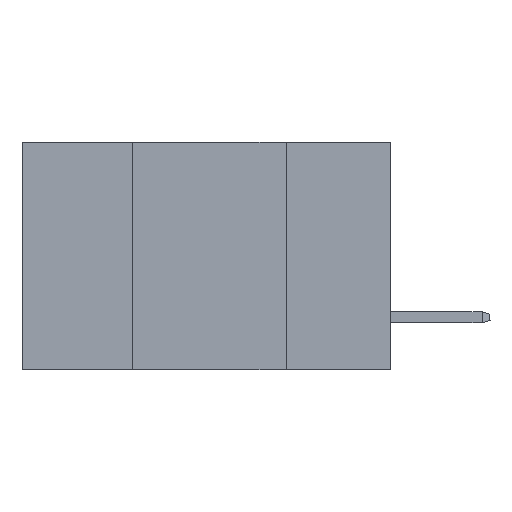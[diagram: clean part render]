
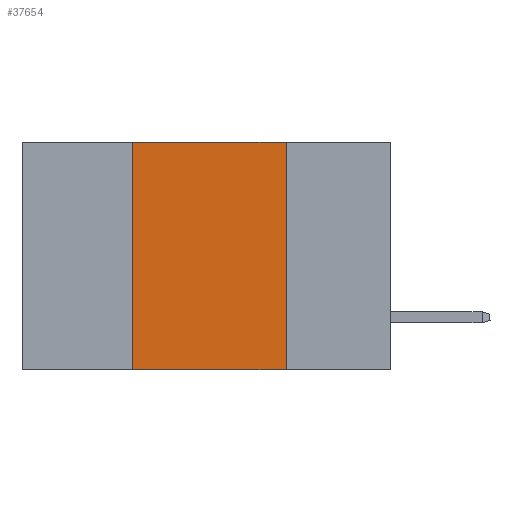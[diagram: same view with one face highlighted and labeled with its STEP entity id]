
A CAD part, left-side view. The second image highlights one B-rep face of the part: STEP entity #37654.
In plain terms, the highlighted planar face has unit normal (-1, 0, 0).
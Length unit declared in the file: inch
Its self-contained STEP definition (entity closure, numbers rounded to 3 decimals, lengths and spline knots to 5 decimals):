
#202 = CARTESIAN_POINT ( 'NONE',  ( 0., 0.17, -0.37 ) ) ;
#1221 = VERTEX_POINT ( 'NONE', #202 ) ;
#5939 = DIRECTION ( 'NONE',  ( 0., 0., 1. ) ) ;
#6066 = CARTESIAN_POINT ( 'NONE',  ( 0., 0.6, 0. ) ) ;
#6353 = LINE ( 'NONE', #49257, #27966 ) ;
#6449 = EDGE_CURVE ( 'NONE', #35542, #47473, #33210, .T. ) ;
#10457 = DIRECTION ( 'NONE',  ( 0., -1., 0. ) ) ;
#10562 = ORIENTED_EDGE ( 'NONE', *, *, #47568, .T. ) ;
#11037 = CARTESIAN_POINT ( 'NONE',  ( 0., 0.17, 0. ) ) ;
#11211 = LINE ( 'NONE', #21221, #14198 ) ;
#11375 = VECTOR ( 'NONE', #35170, 39.37008 ) ;
#12091 = CARTESIAN_POINT ( 'NONE',  ( 0., 0.6, 0. ) ) ;
#14198 = VECTOR ( 'NONE', #5939, 39.37008 ) ;
#19165 = DIRECTION ( 'NONE',  ( 0., 0., -1. ) ) ;
#20255 = ORIENTED_EDGE ( 'NONE', *, *, #38541, .F. ) ;
#21221 = CARTESIAN_POINT ( 'NONE',  ( 0., 0.42, 0. ) ) ;
#21291 = VERTEX_POINT ( 'NONE', #42671 ) ;
#22385 = VECTOR ( 'NONE', #10457, 39.37008 ) ;
#23491 = ORIENTED_EDGE ( 'NONE', *, *, #43522, .F. ) ;
#25007 = ORIENTED_EDGE ( 'NONE', *, *, #6449, .F. ) ;
#27966 = VECTOR ( 'NONE', #19165, 39.37008 ) ;
#30527 = EDGE_LOOP ( 'NONE', ( #23491, #25007, #20255, #10562 ) ) ;
#31194 = PLANE ( 'NONE',  #43829 ) ;
#31625 = CARTESIAN_POINT ( 'NONE',  ( 0., 0.6, -0.37 ) ) ;
#33210 = LINE ( 'NONE', #6066, #22385 ) ;
#33578 = LINE ( 'NONE', #31625, #11375 ) ;
#35170 = DIRECTION ( 'NONE',  ( 0., -1., 0. ) ) ;
#35542 = VERTEX_POINT ( 'NONE', #44096 ) ;
#37654 = ADVANCED_FACE ( 'NONE', ( #49758 ), #31194, .F. ) ;
#38541 = EDGE_CURVE ( 'NONE', #21291, #35542, #11211, .T. ) ;
#38751 = DIRECTION ( 'NONE',  ( 0., 0., -1. ) ) ;
#42671 = CARTESIAN_POINT ( 'NONE',  ( 0., 0.42, -0.37 ) ) ;
#43522 = EDGE_CURVE ( 'NONE', #47473, #1221, #6353, .T. ) ;
#43829 = AXIS2_PLACEMENT_3D ( 'NONE', #12091, #46997, #38751 ) ;
#44096 = CARTESIAN_POINT ( 'NONE',  ( 0., 0.42, 0. ) ) ;
#46997 = DIRECTION ( 'NONE',  ( 1., 0., 0. ) ) ;
#47473 = VERTEX_POINT ( 'NONE', #11037 ) ;
#47568 = EDGE_CURVE ( 'NONE', #21291, #1221, #33578, .T. ) ;
#49257 = CARTESIAN_POINT ( 'NONE',  ( 0., 0.17, 0. ) ) ;
#49758 = FACE_OUTER_BOUND ( 'NONE', #30527, .T. ) ;
